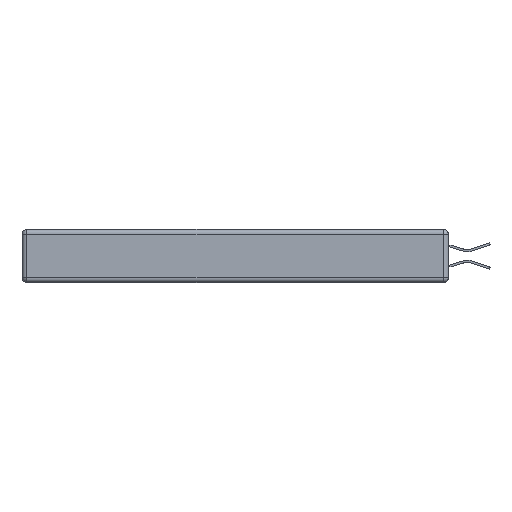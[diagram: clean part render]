
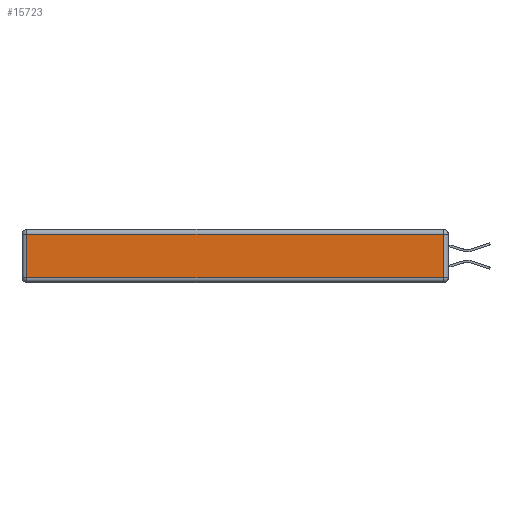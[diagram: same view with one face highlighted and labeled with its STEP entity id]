
A CAD part, left-side view. The second image highlights one B-rep face of the part: STEP entity #15723.
In plain terms, the highlighted planar face has unit normal (-1, 0, 0).
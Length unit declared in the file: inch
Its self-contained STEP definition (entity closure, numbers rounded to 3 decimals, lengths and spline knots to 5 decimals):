
#186 = FACE_OUTER_BOUND ( 'NONE', #5975, .T. ) ;
#761 = DIRECTION ( 'NONE',  ( 0., 1., 0. ) ) ;
#991 = CARTESIAN_POINT ( 'NONE',  ( 0., 2.75, -0.03 ) ) ;
#1182 = VERTEX_POINT ( 'NONE', #10941 ) ;
#2623 = LINE ( 'NONE', #5463, #15910 ) ;
#3294 = ORIENTED_EDGE ( 'NONE', *, *, #14339, .T. ) ;
#3417 = ORIENTED_EDGE ( 'NONE', *, *, #21316, .T. ) ;
#3522 = PLANE ( 'NONE',  #11776 ) ;
#4843 = VECTOR ( 'NONE', #21158, 39.37008 ) ;
#5463 = CARTESIAN_POINT ( 'NONE',  ( 0., 0.03, -0.343 ) ) ;
#5824 = EDGE_CURVE ( 'NONE', #7525, #1182, #16264, .T. ) ;
#5975 = EDGE_LOOP ( 'NONE', ( #15340, #3417, #3294, #22688 ) ) ;
#6236 = CARTESIAN_POINT ( 'NONE',  ( 0., 0.03, -0.03 ) ) ;
#6506 = CARTESIAN_POINT ( 'NONE',  ( 0., 0., -0.313 ) ) ;
#7218 = CARTESIAN_POINT ( 'NONE',  ( 0., 2.72, -0.343 ) ) ;
#7360 = DIRECTION ( 'NONE',  ( 0., 0., 1. ) ) ;
#7525 = VERTEX_POINT ( 'NONE', #17026 ) ;
#7886 = EDGE_CURVE ( 'NONE', #9357, #7525, #14226, .T. ) ;
#9357 = VERTEX_POINT ( 'NONE', #10749 ) ;
#10172 = LINE ( 'NONE', #991, #19889 ) ;
#10749 = CARTESIAN_POINT ( 'NONE',  ( 0., 2.72, -0.03 ) ) ;
#10941 = CARTESIAN_POINT ( 'NONE',  ( 0., 0.03, -0.313 ) ) ;
#11776 = AXIS2_PLACEMENT_3D ( 'NONE', #19610, #12632, #7360 ) ;
#12632 = DIRECTION ( 'NONE',  ( -1., 0., 0. ) ) ;
#14226 = LINE ( 'NONE', #7218, #4843 ) ;
#14339 = EDGE_CURVE ( 'NONE', #20153, #9357, #10172, .T. ) ;
#15340 = ORIENTED_EDGE ( 'NONE', *, *, #5824, .T. ) ;
#15723 = ADVANCED_FACE ( 'NONE', ( #186 ), #3522, .T. ) ;
#15910 = VECTOR ( 'NONE', #18073, 39.37008 ) ;
#16264 = LINE ( 'NONE', #6506, #17688 ) ;
#17026 = CARTESIAN_POINT ( 'NONE',  ( 0., 2.72, -0.313 ) ) ;
#17628 = DIRECTION ( 'NONE',  ( 0., -1., 0. ) ) ;
#17688 = VECTOR ( 'NONE', #17628, 39.37008 ) ;
#18073 = DIRECTION ( 'NONE',  ( 0., 0., 1. ) ) ;
#19610 = CARTESIAN_POINT ( 'NONE',  ( 0., 0., -0.343 ) ) ;
#19889 = VECTOR ( 'NONE', #761, 39.37008 ) ;
#20153 = VERTEX_POINT ( 'NONE', #6236 ) ;
#21158 = DIRECTION ( 'NONE',  ( 0., 0., -1. ) ) ;
#21316 = EDGE_CURVE ( 'NONE', #1182, #20153, #2623, .T. ) ;
#22688 = ORIENTED_EDGE ( 'NONE', *, *, #7886, .T. ) ;
